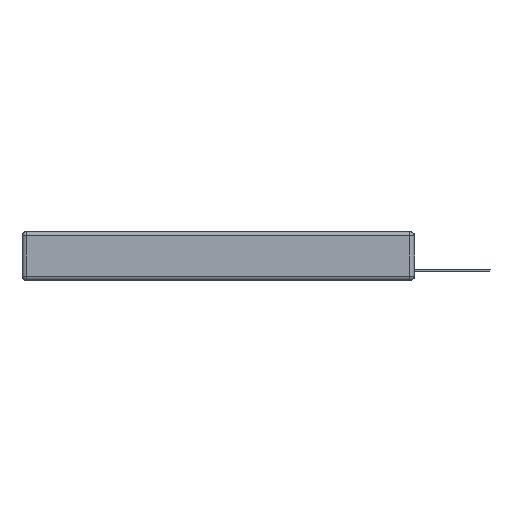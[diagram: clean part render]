
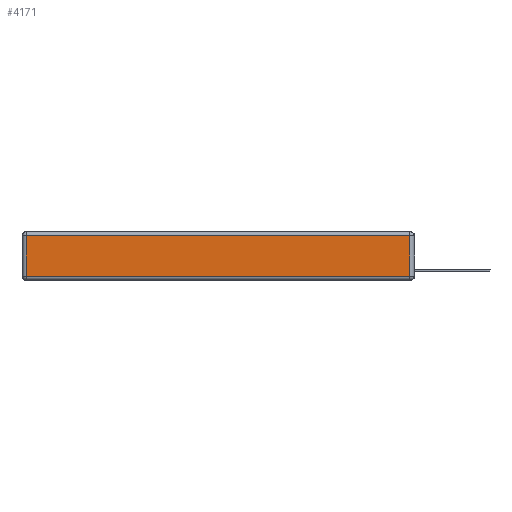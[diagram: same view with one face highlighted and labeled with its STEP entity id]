
A CAD part, left-side view. The second image highlights one B-rep face of the part: STEP entity #4171.
In plain terms, the highlighted planar face has unit normal (-1, 0, 0).
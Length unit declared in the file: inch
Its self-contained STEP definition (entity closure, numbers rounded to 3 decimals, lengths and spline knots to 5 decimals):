
#1022 = LINE ( 'NONE', #9148, #22935 ) ;
#1251 = CARTESIAN_POINT ( 'NONE',  ( 0., 0.03, -0.313 ) ) ;
#1303 = VERTEX_POINT ( 'NONE', #1251 ) ;
#1902 = CARTESIAN_POINT ( 'NONE',  ( 0., 0.03, -0.03 ) ) ;
#2375 = VERTEX_POINT ( 'NONE', #12716 ) ;
#2712 = FACE_OUTER_BOUND ( 'NONE', #3725, .T. ) ;
#3725 = EDGE_LOOP ( 'NONE', ( #20170, #10400, #19241, #8899 ) ) ;
#3856 = AXIS2_PLACEMENT_3D ( 'NONE', #18793, #16937, #8710 ) ;
#4171 = ADVANCED_FACE ( 'NONE', ( #2712 ), #8842, .T. ) ;
#7638 = VECTOR ( 'NONE', #21166, 39.37008 ) ;
#8402 = VERTEX_POINT ( 'NONE', #1902 ) ;
#8710 = DIRECTION ( 'NONE',  ( 0., 0., 1. ) ) ;
#8842 = PLANE ( 'NONE',  #3856 ) ;
#8899 = ORIENTED_EDGE ( 'NONE', *, *, #9268, .T. ) ;
#9148 = CARTESIAN_POINT ( 'NONE',  ( 0., 0.03, -0.343 ) ) ;
#9268 = EDGE_CURVE ( 'NONE', #2375, #11428, #21323, .T. ) ;
#10400 = ORIENTED_EDGE ( 'NONE', *, *, #22620, .T. ) ;
#10936 = CARTESIAN_POINT ( 'NONE',  ( 0., 2.75, -0.03 ) ) ;
#11124 = DIRECTION ( 'NONE',  ( 0., -1., 0. ) ) ;
#11428 = VERTEX_POINT ( 'NONE', #19374 ) ;
#12716 = CARTESIAN_POINT ( 'NONE',  ( 0., 2.72, -0.03 ) ) ;
#12736 = LINE ( 'NONE', #16727, #19303 ) ;
#15759 = EDGE_CURVE ( 'NONE', #11428, #1303, #12736, .T. ) ;
#16727 = CARTESIAN_POINT ( 'NONE',  ( 0., 0., -0.313 ) ) ;
#16937 = DIRECTION ( 'NONE',  ( -1., 0., 0. ) ) ;
#17244 = DIRECTION ( 'NONE',  ( 0., 0., 1. ) ) ;
#18793 = CARTESIAN_POINT ( 'NONE',  ( 0., 0., -0.343 ) ) ;
#19241 = ORIENTED_EDGE ( 'NONE', *, *, #20388, .T. ) ;
#19283 = LINE ( 'NONE', #10936, #7638 ) ;
#19303 = VECTOR ( 'NONE', #11124, 39.37008 ) ;
#19374 = CARTESIAN_POINT ( 'NONE',  ( 0., 2.72, -0.313 ) ) ;
#19682 = VECTOR ( 'NONE', #23570, 39.37008 ) ;
#20170 = ORIENTED_EDGE ( 'NONE', *, *, #15759, .T. ) ;
#20388 = EDGE_CURVE ( 'NONE', #8402, #2375, #19283, .T. ) ;
#21166 = DIRECTION ( 'NONE',  ( 0., 1., 0. ) ) ;
#21323 = LINE ( 'NONE', #23700, #19682 ) ;
#22620 = EDGE_CURVE ( 'NONE', #1303, #8402, #1022, .T. ) ;
#22935 = VECTOR ( 'NONE', #17244, 39.37008 ) ;
#23570 = DIRECTION ( 'NONE',  ( 0., 0., -1. ) ) ;
#23700 = CARTESIAN_POINT ( 'NONE',  ( 0., 2.72, -0.343 ) ) ;
